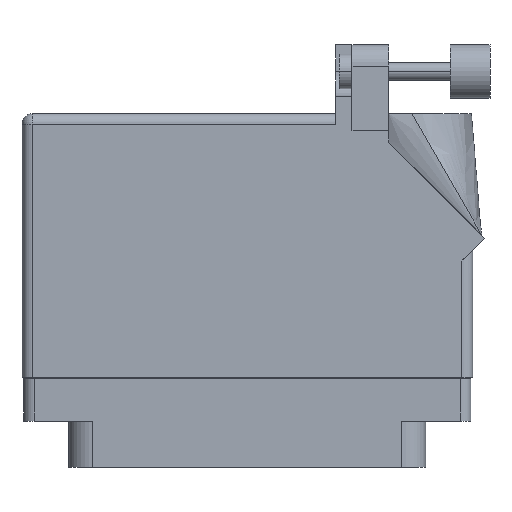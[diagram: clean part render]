
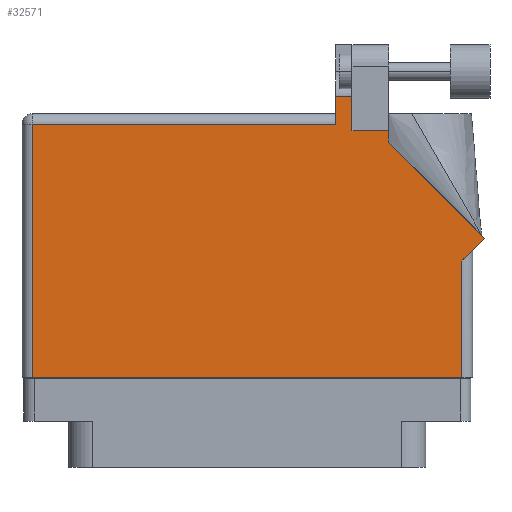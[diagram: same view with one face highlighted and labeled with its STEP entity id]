
A CAD part, front view. The second image highlights one B-rep face of the part: STEP entity #32571.
In plain terms, the highlighted face is planar.
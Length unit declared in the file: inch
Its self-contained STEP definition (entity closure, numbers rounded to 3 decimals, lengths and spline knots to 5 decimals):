
#819 = CARTESIAN_POINT ( 'NONE',  ( 0.82, 1.33, 0.455 ) ) ;
#1173 = VERTEX_POINT ( 'NONE', #7402 ) ;
#1260 = VECTOR ( 'NONE', #37210, 39.37008 ) ;
#1318 = CARTESIAN_POINT ( 'NONE',  ( 1.244, 0.637, 0.455 ) ) ;
#2829 = LINE ( 'NONE', #819, #28769 ) ;
#4657 = CARTESIAN_POINT ( 'NONE',  ( -1.306, -0.1, 0.455 ) ) ;
#5364 = VERTEX_POINT ( 'NONE', #22167 ) ;
#6192 = ORIENTED_EDGE ( 'NONE', *, *, #21018, .T. ) ;
#6244 = AXIS2_PLACEMENT_3D ( 'NONE', #16002, #43023, #12642 ) ;
#7078 = LINE ( 'NONE', #27425, #17530 ) ;
#7402 = CARTESIAN_POINT ( 'NONE',  ( 1.37671, 0.70771, 0.455 ) ) ;
#7528 = DIRECTION ( 'NONE',  ( 0., -1., 0. ) ) ;
#7561 = ORIENTED_EDGE ( 'NONE', *, *, #42411, .T. ) ;
#7795 = ORIENTED_EDGE ( 'NONE', *, *, #39348, .T. ) ;
#8156 = DIRECTION ( 'NONE',  ( 0., 1., 0. ) ) ;
#8467 = LINE ( 'NONE', #1318, #37981 ) ;
#8870 = EDGE_LOOP ( 'NONE', ( #14560, #27138, #37096, #35764, #13624, #7561, #10208, #7795, #6192, #22294, #39088 ) ) ;
#10208 = ORIENTED_EDGE ( 'NONE', *, *, #15155, .T. ) ;
#10759 = VECTOR ( 'NONE', #21357, 39.37008 ) ;
#11156 = VERTEX_POINT ( 'NONE', #31196 ) ;
#11722 = EDGE_CURVE ( 'NONE', #5364, #39062, #12391, .T. ) ;
#11836 = LINE ( 'NONE', #40447, #1260 ) ;
#12314 = CARTESIAN_POINT ( 'NONE',  ( -1.244, 1.368, 0.455 ) ) ;
#12391 = LINE ( 'NONE', #38474, #28791 ) ;
#12426 = VERTEX_POINT ( 'NONE', #34397 ) ;
#12642 = DIRECTION ( 'NONE',  ( -1., 0., 0. ) ) ;
#13624 = ORIENTED_EDGE ( 'NONE', *, *, #40904, .T. ) ;
#13728 = CARTESIAN_POINT ( 'NONE',  ( 0.513, 1.368, 0.455 ) ) ;
#14119 = CARTESIAN_POINT ( 'NONE',  ( -1.244, -0.1, 0.455 ) ) ;
#14175 = EDGE_CURVE ( 'NONE', #24623, #38154, #36265, .T. ) ;
#14560 = ORIENTED_EDGE ( 'NONE', *, *, #14175, .T. ) ;
#14816 = DIRECTION ( 'NONE',  ( 1., 0., 0. ) ) ;
#14921 = VECTOR ( 'NONE', #14816, 39.37008 ) ;
#15155 = EDGE_CURVE ( 'NONE', #11156, #27389, #8467, .T. ) ;
#16002 = CARTESIAN_POINT ( 'NONE',  ( -1.306, 1.43, 0.455 ) ) ;
#17530 = VECTOR ( 'NONE', #30683, 39.37008 ) ;
#17609 = EDGE_CURVE ( 'NONE', #39062, #36981, #7078, .T. ) ;
#20920 = EDGE_CURVE ( 'NONE', #12426, #24623, #2829, .T. ) ;
#21018 = EDGE_CURVE ( 'NONE', #1173, #39044, #38205, .T. ) ;
#21149 = CARTESIAN_POINT ( 'NONE',  ( 0.93777, 1.5315, 0.455 ) ) ;
#21357 = DIRECTION ( 'NONE',  ( -0.707, 0.707, 0. ) ) ;
#21802 = EDGE_CURVE ( 'NONE', #38154, #5364, #29665, .T. ) ;
#22167 = CARTESIAN_POINT ( 'NONE',  ( 0.513, 1.5315, 0.455 ) ) ;
#22294 = ORIENTED_EDGE ( 'NONE', *, *, #41624, .T. ) ;
#22468 = LINE ( 'NONE', #14119, #30923 ) ;
#22515 = CARTESIAN_POINT ( 'NONE',  ( 0.607, 1.33, 0.455 ) ) ;
#22556 = VECTOR ( 'NONE', #39270, 39.37008 ) ;
#23493 = FACE_OUTER_BOUND ( 'NONE', #8870, .T. ) ;
#23749 = CARTESIAN_POINT ( 'NONE',  ( 1.244, 0.575, 0.455 ) ) ;
#24239 = DIRECTION ( 'NONE',  ( -1., 0., 0. ) ) ;
#24623 = VERTEX_POINT ( 'NONE', #33836 ) ;
#25243 = DIRECTION ( 'NONE',  ( 0., -1., 0. ) ) ;
#26223 = PLANE ( 'NONE',  #6244 ) ;
#27138 = ORIENTED_EDGE ( 'NONE', *, *, #21802, .T. ) ;
#27389 = VERTEX_POINT ( 'NONE', #23749 ) ;
#27425 = CARTESIAN_POINT ( 'NONE',  ( -1.306, 1.368, 0.455 ) ) ;
#28769 = VECTOR ( 'NONE', #31256, 39.37008 ) ;
#28791 = VECTOR ( 'NONE', #25243, 39.37008 ) ;
#29535 = DIRECTION ( 'NONE',  ( 0.707, 0.707, 0. ) ) ;
#29665 = LINE ( 'NONE', #21149, #40698 ) ;
#29710 = LINE ( 'NONE', #4657, #14921 ) ;
#30490 = VECTOR ( 'NONE', #29535, 39.37008 ) ;
#30683 = DIRECTION ( 'NONE',  ( -1., 0., 0. ) ) ;
#30923 = VECTOR ( 'NONE', #7528, 39.37008 ) ;
#31196 = CARTESIAN_POINT ( 'NONE',  ( 1.244, -0.1, 0.455 ) ) ;
#31256 = DIRECTION ( 'NONE',  ( -1., 0., 0. ) ) ;
#32298 = CARTESIAN_POINT ( 'NONE',  ( 1.37671, 0.70771, 0.455 ) ) ;
#32571 = ADVANCED_FACE ( 'NONE', ( #23493 ), #26223, .F. ) ;
#33204 = CARTESIAN_POINT ( 'NONE',  ( 0.607, 1.5315, 0.455 ) ) ;
#33836 = CARTESIAN_POINT ( 'NONE',  ( 0.607, 1.33, 0.455 ) ) ;
#34397 = CARTESIAN_POINT ( 'NONE',  ( 0.82, 1.33, 0.455 ) ) ;
#35425 = CARTESIAN_POINT ( 'NONE',  ( 1.306, 0.637, 0.455 ) ) ;
#35764 = ORIENTED_EDGE ( 'NONE', *, *, #17609, .T. ) ;
#36265 = LINE ( 'NONE', #22515, #22556 ) ;
#36981 = VERTEX_POINT ( 'NONE', #12314 ) ;
#37096 = ORIENTED_EDGE ( 'NONE', *, *, #11722, .T. ) ;
#37210 = DIRECTION ( 'NONE',  ( 0., 1., 0. ) ) ;
#37981 = VECTOR ( 'NONE', #8156, 39.37008 ) ;
#38154 = VERTEX_POINT ( 'NONE', #33204 ) ;
#38205 = LINE ( 'NONE', #32298, #10759 ) ;
#38474 = CARTESIAN_POINT ( 'NONE',  ( 0.513, 1.43, 0.455 ) ) ;
#39044 = VERTEX_POINT ( 'NONE', #40717 ) ;
#39062 = VERTEX_POINT ( 'NONE', #13728 ) ;
#39088 = ORIENTED_EDGE ( 'NONE', *, *, #20920, .T. ) ;
#39270 = DIRECTION ( 'NONE',  ( 0., 1., 0. ) ) ;
#39348 = EDGE_CURVE ( 'NONE', #27389, #1173, #39931, .T. ) ;
#39637 = CARTESIAN_POINT ( 'NONE',  ( -1.244, -0.1, 0.455 ) ) ;
#39931 = LINE ( 'NONE', #35425, #30490 ) ;
#40447 = CARTESIAN_POINT ( 'NONE',  ( 0.82, 1.26442, 0.455 ) ) ;
#40698 = VECTOR ( 'NONE', #24239, 39.37008 ) ;
#40717 = CARTESIAN_POINT ( 'NONE',  ( 0.82, 1.26442, 0.455 ) ) ;
#40904 = EDGE_CURVE ( 'NONE', #36981, #43219, #22468, .T. ) ;
#41624 = EDGE_CURVE ( 'NONE', #39044, #12426, #11836, .T. ) ;
#42411 = EDGE_CURVE ( 'NONE', #43219, #11156, #29710, .T. ) ;
#43023 = DIRECTION ( 'NONE',  ( 0., 0., -1. ) ) ;
#43219 = VERTEX_POINT ( 'NONE', #39637 ) ;
